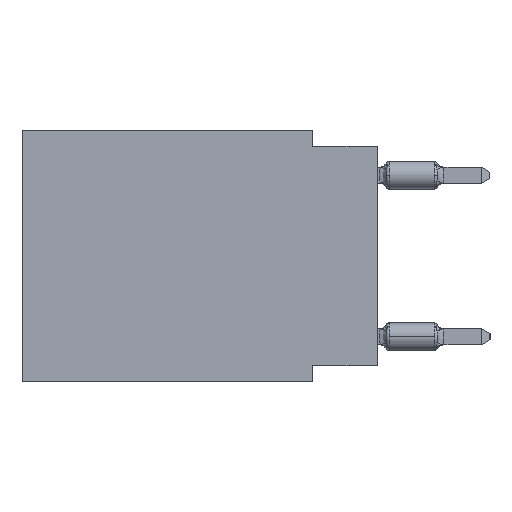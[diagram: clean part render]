
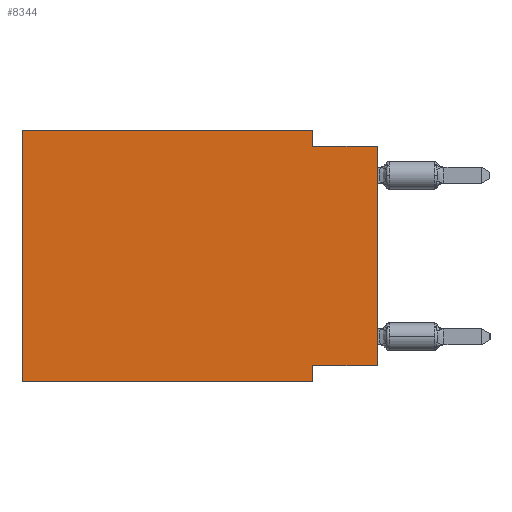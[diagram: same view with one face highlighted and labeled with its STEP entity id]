
A CAD part, left-side view. The second image highlights one B-rep face of the part: STEP entity #8344.
In plain terms, the highlighted planar face has unit normal (-1, 0, 0).
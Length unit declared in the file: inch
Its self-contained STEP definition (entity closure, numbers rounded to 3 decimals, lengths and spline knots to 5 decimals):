
#737 = ORIENTED_EDGE ( 'NONE', *, *, #17853, .F. ) ;
#797 = CARTESIAN_POINT ( 'NONE',  ( 0., 0., -0.365 ) ) ;
#813 = EDGE_CURVE ( 'NONE', #19088, #19586, #8490, .T. ) ;
#880 = LINE ( 'NONE', #5741, #16989 ) ;
#1542 = EDGE_CURVE ( 'NONE', #14893, #19849, #15842, .T. ) ;
#1807 = CARTESIAN_POINT ( 'NONE',  ( 0., 0.55, -0.39 ) ) ;
#2516 = VERTEX_POINT ( 'NONE', #19402 ) ;
#3697 = VECTOR ( 'NONE', #13308, 39.37008 ) ;
#3768 = ORIENTED_EDGE ( 'NONE', *, *, #9664, .F. ) ;
#4695 = VECTOR ( 'NONE', #5437, 39.37008 ) ;
#4807 = ORIENTED_EDGE ( 'NONE', *, *, #813, .F. ) ;
#4906 = DIRECTION ( 'NONE',  ( 0., -1., 0. ) ) ;
#4954 = AXIS2_PLACEMENT_3D ( 'NONE', #14068, #12625, #7803 ) ;
#4983 = CARTESIAN_POINT ( 'NONE',  ( 0., 0., -0.025 ) ) ;
#5100 = ORIENTED_EDGE ( 'NONE', *, *, #11315, .F. ) ;
#5437 = DIRECTION ( 'NONE',  ( 0., 0., 1. ) ) ;
#5741 = CARTESIAN_POINT ( 'NONE',  ( 0., 0.55, 0. ) ) ;
#6311 = ORIENTED_EDGE ( 'NONE', *, *, #1542, .F. ) ;
#6745 = CARTESIAN_POINT ( 'NONE',  ( 0., 0.1, 0. ) ) ;
#6750 = VECTOR ( 'NONE', #11600, 39.37008 ) ;
#6790 = CARTESIAN_POINT ( 'NONE',  ( 0., 0.1, -0.39 ) ) ;
#7534 = VECTOR ( 'NONE', #12882, 39.37008 ) ;
#7555 = LINE ( 'NONE', #10567, #17418 ) ;
#7651 = CARTESIAN_POINT ( 'NONE',  ( 0., 0.55, 0. ) ) ;
#7803 = DIRECTION ( 'NONE',  ( 0., 0., -1. ) ) ;
#7975 = LINE ( 'NONE', #6745, #7534 ) ;
#8344 = ADVANCED_FACE ( 'NONE', ( #14165 ), #18521, .F. ) ;
#8424 = VECTOR ( 'NONE', #19072, 39.37008 ) ;
#8490 = LINE ( 'NONE', #797, #3697 ) ;
#8702 = VERTEX_POINT ( 'NONE', #12675 ) ;
#8896 = CARTESIAN_POINT ( 'NONE',  ( 0., 0., -0.365 ) ) ;
#9252 = ORIENTED_EDGE ( 'NONE', *, *, #12511, .T. ) ;
#9664 = EDGE_CURVE ( 'NONE', #19586, #8702, #19221, .T. ) ;
#10469 = CARTESIAN_POINT ( 'NONE',  ( 0., 0.1, -0.365 ) ) ;
#10482 = CARTESIAN_POINT ( 'NONE',  ( 0., 0., -0.025 ) ) ;
#10567 = CARTESIAN_POINT ( 'NONE',  ( 0., 0.55, -0.39 ) ) ;
#11315 = EDGE_CURVE ( 'NONE', #2516, #11974, #14104, .T. ) ;
#11571 = EDGE_LOOP ( 'NONE', ( #9252, #5100, #737, #17939, #6311, #14277, #3768, #4807 ) ) ;
#11600 = DIRECTION ( 'NONE',  ( 0., 0., -1. ) ) ;
#11974 = VERTEX_POINT ( 'NONE', #4983 ) ;
#12511 = EDGE_CURVE ( 'NONE', #19088, #11974, #14937, .T. ) ;
#12625 = DIRECTION ( 'NONE',  ( 1., 0., 0. ) ) ;
#12675 = CARTESIAN_POINT ( 'NONE',  ( 0., 0.1, -0.39 ) ) ;
#12882 = DIRECTION ( 'NONE',  ( 0., 0., -1. ) ) ;
#13101 = DIRECTION ( 'NONE',  ( 0., -1., 0. ) ) ;
#13308 = DIRECTION ( 'NONE',  ( 0., 1., 0. ) ) ;
#13593 = DIRECTION ( 'NONE',  ( 0., -1., 0. ) ) ;
#13661 = EDGE_CURVE ( 'NONE', #19849, #18491, #880, .T. ) ;
#14068 = CARTESIAN_POINT ( 'NONE',  ( 0., 0.55, 0. ) ) ;
#14104 = LINE ( 'NONE', #10482, #15309 ) ;
#14165 = FACE_OUTER_BOUND ( 'NONE', #11571, .T. ) ;
#14277 = ORIENTED_EDGE ( 'NONE', *, *, #15108, .T. ) ;
#14684 = CARTESIAN_POINT ( 'NONE',  ( 0., 0.1, 0. ) ) ;
#14893 = VERTEX_POINT ( 'NONE', #1807 ) ;
#14937 = LINE ( 'NONE', #18080, #4695 ) ;
#15108 = EDGE_CURVE ( 'NONE', #14893, #8702, #7555, .T. ) ;
#15309 = VECTOR ( 'NONE', #4906, 39.37008 ) ;
#15842 = LINE ( 'NONE', #7651, #8424 ) ;
#16989 = VECTOR ( 'NONE', #13101, 39.37008 ) ;
#17418 = VECTOR ( 'NONE', #13593, 39.37008 ) ;
#17853 = EDGE_CURVE ( 'NONE', #18491, #2516, #7975, .T. ) ;
#17939 = ORIENTED_EDGE ( 'NONE', *, *, #13661, .F. ) ;
#18080 = CARTESIAN_POINT ( 'NONE',  ( 0., 0., 0. ) ) ;
#18491 = VERTEX_POINT ( 'NONE', #14684 ) ;
#18521 = PLANE ( 'NONE',  #4954 ) ;
#19072 = DIRECTION ( 'NONE',  ( 0., 0., 1. ) ) ;
#19088 = VERTEX_POINT ( 'NONE', #8896 ) ;
#19221 = LINE ( 'NONE', #6790, #6750 ) ;
#19402 = CARTESIAN_POINT ( 'NONE',  ( 0., 0.1, -0.025 ) ) ;
#19586 = VERTEX_POINT ( 'NONE', #10469 ) ;
#19753 = CARTESIAN_POINT ( 'NONE',  ( 0., 0.55, 0. ) ) ;
#19849 = VERTEX_POINT ( 'NONE', #19753 ) ;
